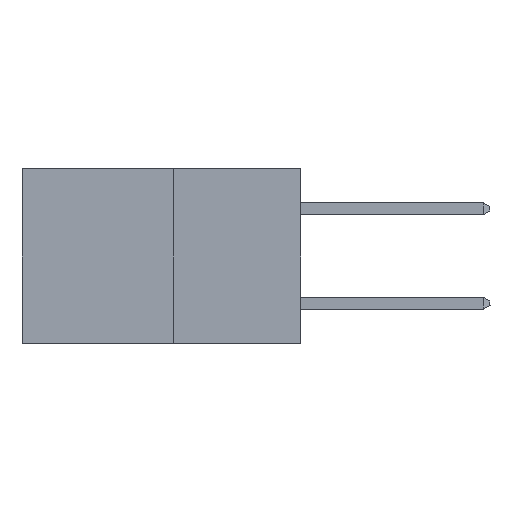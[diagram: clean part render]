
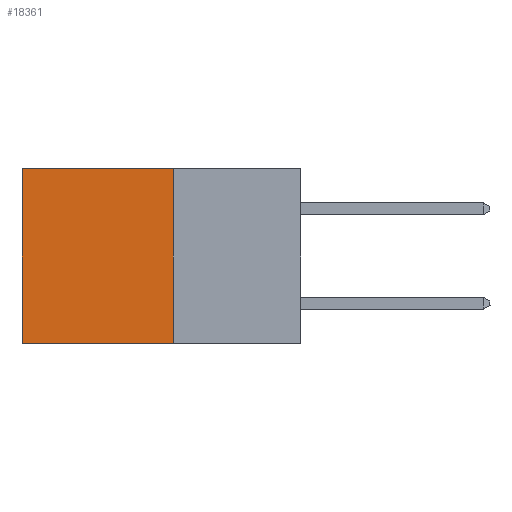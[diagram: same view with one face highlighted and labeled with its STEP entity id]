
A CAD part, left-side view. The second image highlights one B-rep face of the part: STEP entity #18361.
In plain terms, the highlighted planar face has unit normal (-1, 0, 0).
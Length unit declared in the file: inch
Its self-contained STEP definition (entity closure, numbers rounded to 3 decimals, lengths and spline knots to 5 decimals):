
#335 = CARTESIAN_POINT ( 'NONE',  ( 0.277, 0.27, 0. ) ) ;
#891 = DIRECTION ( 'NONE',  ( 1., 0., 0. ) ) ;
#1694 = CARTESIAN_POINT ( 'NONE',  ( 0.277, 0.59, -0.37 ) ) ;
#2236 = CARTESIAN_POINT ( 'NONE',  ( 0.277, 0.59, 0. ) ) ;
#2757 = ORIENTED_EDGE ( 'NONE', *, *, #14914, .F. ) ;
#3252 = CARTESIAN_POINT ( 'NONE',  ( 0.277, 0.59, -0.37 ) ) ;
#7769 = DIRECTION ( 'NONE',  ( 0., 0., -1. ) ) ;
#8026 = VECTOR ( 'NONE', #20523, 39.37008 ) ;
#8493 = VERTEX_POINT ( 'NONE', #11057 ) ;
#9915 = DIRECTION ( 'NONE',  ( 0., 1., 0. ) ) ;
#10170 = PLANE ( 'NONE',  #13423 ) ;
#10551 = VECTOR ( 'NONE', #17737, 39.37008 ) ;
#11057 = CARTESIAN_POINT ( 'NONE',  ( 0.277, 0.27, -0.37 ) ) ;
#13423 = AXIS2_PLACEMENT_3D ( 'NONE', #14722, #891, #16972 ) ;
#14035 = VERTEX_POINT ( 'NONE', #2236 ) ;
#14330 = VERTEX_POINT ( 'NONE', #3252 ) ;
#14722 = CARTESIAN_POINT ( 'NONE',  ( 0.277, 0.27, -0.37 ) ) ;
#14849 = EDGE_CURVE ( 'NONE', #21477, #14035, #24736, .T. ) ;
#14914 = EDGE_CURVE ( 'NONE', #21477, #8493, #29305, .T. ) ;
#16972 = DIRECTION ( 'NONE',  ( 0., 0., -1. ) ) ;
#17210 = ORIENTED_EDGE ( 'NONE', *, *, #14849, .T. ) ;
#17737 = DIRECTION ( 'NONE',  ( 0., 0., -1. ) ) ;
#17962 = LINE ( 'NONE', #1694, #10551 ) ;
#18274 = CARTESIAN_POINT ( 'NONE',  ( 0.277, 0.27, -0.37 ) ) ;
#18361 = ADVANCED_FACE ( 'NONE', ( #23055 ), #10170, .F. ) ;
#18790 = VECTOR ( 'NONE', #9915, 39.37008 ) ;
#18937 = CARTESIAN_POINT ( 'NONE',  ( 0.277, 0.27, 0. ) ) ;
#19852 = ORIENTED_EDGE ( 'NONE', *, *, #25769, .T. ) ;
#20523 = DIRECTION ( 'NONE',  ( 0., 1., 0. ) ) ;
#21374 = CARTESIAN_POINT ( 'NONE',  ( 0.277, 0.27, -0.37 ) ) ;
#21477 = VERTEX_POINT ( 'NONE', #335 ) ;
#23055 = FACE_OUTER_BOUND ( 'NONE', #23168, .T. ) ;
#23168 = EDGE_LOOP ( 'NONE', ( #19852, #25644, #2757, #17210 ) ) ;
#23340 = VECTOR ( 'NONE', #7769, 39.37008 ) ;
#24736 = LINE ( 'NONE', #18937, #18790 ) ;
#25244 = EDGE_CURVE ( 'NONE', #8493, #14330, #25375, .T. ) ;
#25375 = LINE ( 'NONE', #18274, #8026 ) ;
#25644 = ORIENTED_EDGE ( 'NONE', *, *, #25244, .F. ) ;
#25769 = EDGE_CURVE ( 'NONE', #14035, #14330, #17962, .T. ) ;
#29305 = LINE ( 'NONE', #21374, #23340 ) ;
